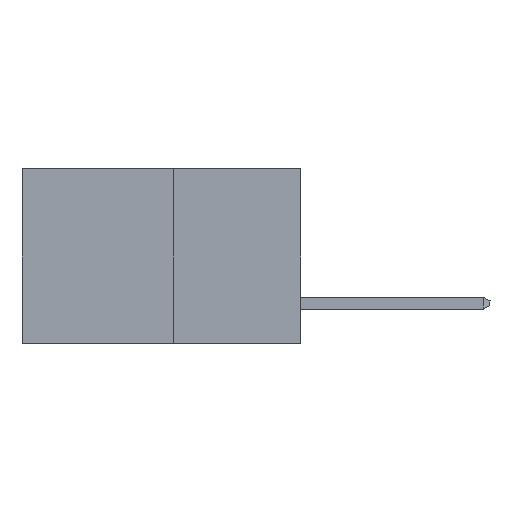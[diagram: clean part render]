
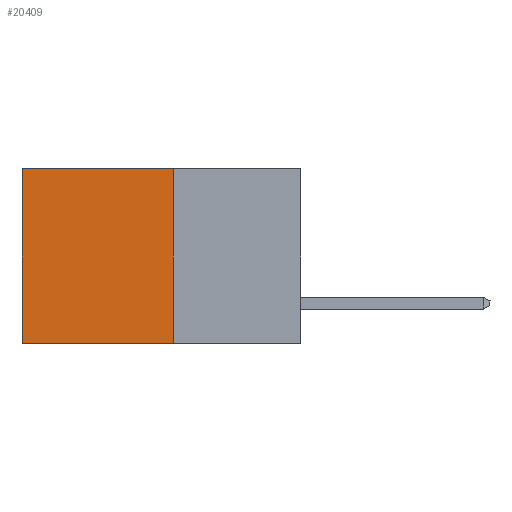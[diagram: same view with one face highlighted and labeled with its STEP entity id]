
A CAD part, left-side view. The second image highlights one B-rep face of the part: STEP entity #20409.
In plain terms, the highlighted planar face has unit normal (-1, 0, 0).
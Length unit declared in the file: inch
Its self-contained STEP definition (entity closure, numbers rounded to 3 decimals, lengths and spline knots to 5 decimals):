
#887 = AXIS2_PLACEMENT_3D ( 'NONE', #22434, #11464, #26891 ) ;
#1087 = ORIENTED_EDGE ( 'NONE', *, *, #21126, .F. ) ;
#1147 = EDGE_LOOP ( 'NONE', ( #6156, #1087, #21188, #4766 ) ) ;
#3923 = VERTEX_POINT ( 'NONE', #17762 ) ;
#4305 = CARTESIAN_POINT ( 'NONE',  ( 0.277, 0.27, -0.37 ) ) ;
#4766 = ORIENTED_EDGE ( 'NONE', *, *, #7101, .T. ) ;
#5693 = FACE_OUTER_BOUND ( 'NONE', #1147, .T. ) ;
#6156 = ORIENTED_EDGE ( 'NONE', *, *, #12198, .T. ) ;
#7075 = CARTESIAN_POINT ( 'NONE',  ( 0.277, 0.27, -0.37 ) ) ;
#7101 = EDGE_CURVE ( 'NONE', #17830, #3923, #27457, .T. ) ;
#7192 = CARTESIAN_POINT ( 'NONE',  ( 0.277, 0.27, 0. ) ) ;
#9057 = VERTEX_POINT ( 'NONE', #4305 ) ;
#9230 = VECTOR ( 'NONE', #12899, 39.37008 ) ;
#10912 = LINE ( 'NONE', #22610, #21915 ) ;
#11464 = DIRECTION ( 'NONE',  ( 1., 0., 0. ) ) ;
#11683 = CARTESIAN_POINT ( 'NONE',  ( 0.277, 0.59, -0.37 ) ) ;
#12198 = EDGE_CURVE ( 'NONE', #3923, #17239, #10912, .T. ) ;
#12899 = DIRECTION ( 'NONE',  ( 0., 1., 0. ) ) ;
#14369 = CARTESIAN_POINT ( 'NONE',  ( 0.277, 0.27, -0.37 ) ) ;
#15643 = VECTOR ( 'NONE', #26860, 39.37008 ) ;
#17239 = VERTEX_POINT ( 'NONE', #11683 ) ;
#17762 = CARTESIAN_POINT ( 'NONE',  ( 0.277, 0.59, 0. ) ) ;
#17830 = VERTEX_POINT ( 'NONE', #7192 ) ;
#19568 = CARTESIAN_POINT ( 'NONE',  ( 0.277, 0.27, 0. ) ) ;
#20409 = ADVANCED_FACE ( 'NONE', ( #5693 ), #26788, .F. ) ;
#21126 = EDGE_CURVE ( 'NONE', #9057, #17239, #28048, .T. ) ;
#21188 = ORIENTED_EDGE ( 'NONE', *, *, #21381, .F. ) ;
#21381 = EDGE_CURVE ( 'NONE', #17830, #9057, #27704, .T. ) ;
#21915 = VECTOR ( 'NONE', #22752, 39.37008 ) ;
#22434 = CARTESIAN_POINT ( 'NONE',  ( 0.277, 0.27, -0.37 ) ) ;
#22610 = CARTESIAN_POINT ( 'NONE',  ( 0.277, 0.59, -0.37 ) ) ;
#22752 = DIRECTION ( 'NONE',  ( 0., 0., -1. ) ) ;
#23375 = DIRECTION ( 'NONE',  ( 0., 0., -1. ) ) ;
#26360 = VECTOR ( 'NONE', #23375, 39.37008 ) ;
#26788 = PLANE ( 'NONE',  #887 ) ;
#26860 = DIRECTION ( 'NONE',  ( 0., 1., 0. ) ) ;
#26891 = DIRECTION ( 'NONE',  ( 0., 0., -1. ) ) ;
#27457 = LINE ( 'NONE', #19568, #9230 ) ;
#27704 = LINE ( 'NONE', #14369, #26360 ) ;
#28048 = LINE ( 'NONE', #7075, #15643 ) ;
